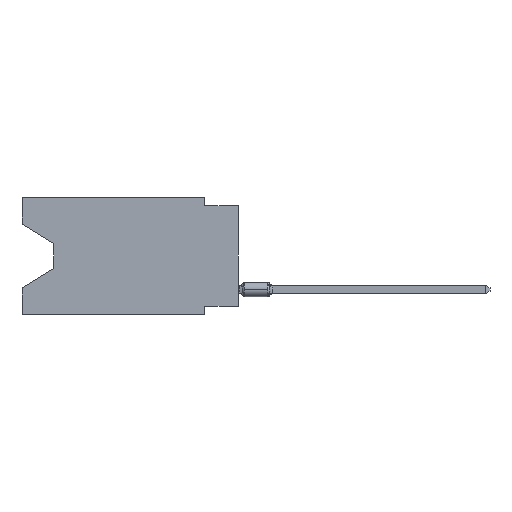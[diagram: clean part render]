
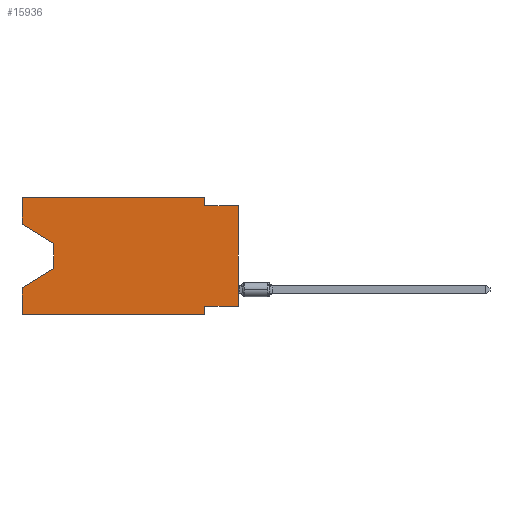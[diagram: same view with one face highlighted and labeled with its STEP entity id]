
A CAD part, left-side view. The second image highlights one B-rep face of the part: STEP entity #15936.
In plain terms, the highlighted planar face has unit normal (-1, 0, 0).
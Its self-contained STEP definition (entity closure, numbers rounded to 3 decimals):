
#45 = CARTESIAN_POINT ( 'NONE',  ( 0., 16.383, -8.89 ) ) ;
#59 = VECTOR ( 'NONE', #18303, 1000. ) ;
#830 = EDGE_CURVE ( 'NONE', #9263, #9711, #10362, .T. ) ;
#850 = LINE ( 'NONE', #15867, #10318 ) ;
#863 = VECTOR ( 'NONE', #14521, 1000. ) ;
#938 = VECTOR ( 'NONE', #13964, 1000. ) ;
#1732 = ORIENTED_EDGE ( 'NONE', *, *, #13332, .F. ) ;
#1753 = VERTEX_POINT ( 'NONE', #17822 ) ;
#1893 = VERTEX_POINT ( 'NONE', #14562 ) ;
#1903 = EDGE_CURVE ( 'NONE', #18999, #1893, #7029, .T. ) ;
#1999 = LINE ( 'NONE', #7998, #16949 ) ;
#2088 = LINE ( 'NONE', #8080, #59 ) ;
#2540 = DIRECTION ( 'NONE',  ( 0., 0., -1. ) ) ;
#2624 = CARTESIAN_POINT ( 'NONE',  ( 0., 0., -8.255 ) ) ;
#3233 = EDGE_LOOP ( 'NONE', ( #17978, #8627, #7239, #8827, #5678, #8044, #18217, #5854, #4483, #6046, #1732, #8704 ) ) ;
#4319 = CARTESIAN_POINT ( 'NONE',  ( 0., 13.97, -5.385 ) ) ;
#4483 = ORIENTED_EDGE ( 'NONE', *, *, #12300, .F. ) ;
#4683 = DIRECTION ( 'NONE',  ( 0., 0., 1. ) ) ;
#4895 = VERTEX_POINT ( 'NONE', #19130 ) ;
#4919 = VECTOR ( 'NONE', #6568, 1000. ) ;
#4926 = EDGE_CURVE ( 'NONE', #18999, #15049, #16763, .T. ) ;
#4992 = CARTESIAN_POINT ( 'NONE',  ( 0., 0., -0.635 ) ) ;
#5051 = LINE ( 'NONE', #5227, #938 ) ;
#5227 = CARTESIAN_POINT ( 'NONE',  ( 0., 2.54, 0. ) ) ;
#5397 = EDGE_CURVE ( 'NONE', #9263, #11819, #1999, .T. ) ;
#5626 = VERTEX_POINT ( 'NONE', #17776 ) ;
#5678 = ORIENTED_EDGE ( 'NONE', *, *, #4926, .T. ) ;
#5681 = VECTOR ( 'NONE', #16667, 1000. ) ;
#5854 = ORIENTED_EDGE ( 'NONE', *, *, #830, .T. ) ;
#6046 = ORIENTED_EDGE ( 'NONE', *, *, #9936, .F. ) ;
#6436 = DIRECTION ( 'NONE',  ( 0., 1., 0. ) ) ;
#6568 = DIRECTION ( 'NONE',  ( 0., -1., 0. ) ) ;
#6731 = DIRECTION ( 'NONE',  ( 0., 0., 1. ) ) ;
#7029 = LINE ( 'NONE', #9866, #13576 ) ;
#7239 = ORIENTED_EDGE ( 'NONE', *, *, #18160, .T. ) ;
#7241 = LINE ( 'NONE', #14965, #12222 ) ;
#7480 = AXIS2_PLACEMENT_3D ( 'NONE', #15069, #14025, #18013 ) ;
#7541 = CARTESIAN_POINT ( 'NONE',  ( 0., 16.383, 0. ) ) ;
#7979 = PLANE ( 'NONE',  #7480 ) ;
#7998 = CARTESIAN_POINT ( 'NONE',  ( 0., 0., -8.255 ) ) ;
#8044 = ORIENTED_EDGE ( 'NONE', *, *, #15213, .F. ) ;
#8080 = CARTESIAN_POINT ( 'NONE',  ( 0., 13.97, -3.505 ) ) ;
#8383 = VERTEX_POINT ( 'NONE', #12619 ) ;
#8545 = VECTOR ( 'NONE', #10458, 1000. ) ;
#8553 = LINE ( 'NONE', #13445, #863 ) ;
#8627 = ORIENTED_EDGE ( 'NONE', *, *, #19151, .T. ) ;
#8704 = ORIENTED_EDGE ( 'NONE', *, *, #9469, .F. ) ;
#8827 = ORIENTED_EDGE ( 'NONE', *, *, #1903, .F. ) ;
#8927 = DIRECTION ( 'NONE',  ( 0., 0.855, -0.519 ) ) ;
#9263 = VERTEX_POINT ( 'NONE', #2624 ) ;
#9469 = EDGE_CURVE ( 'NONE', #8383, #1753, #10583, .T. ) ;
#9711 = VERTEX_POINT ( 'NONE', #17412 ) ;
#9866 = CARTESIAN_POINT ( 'NONE',  ( 0., 16.383, 0. ) ) ;
#9896 = LINE ( 'NONE', #4992, #4919 ) ;
#9936 = EDGE_CURVE ( 'NONE', #18214, #4895, #5051, .T. ) ;
#10318 = VECTOR ( 'NONE', #2540, 1000. ) ;
#10362 = LINE ( 'NONE', #13372, #8545 ) ;
#10385 = DIRECTION ( 'NONE',  ( 0., -0.855, -0.519 ) ) ;
#10416 = LINE ( 'NONE', #16381, #18212 ) ;
#10458 = DIRECTION ( 'NONE',  ( 0., 0., 1. ) ) ;
#10583 = LINE ( 'NONE', #7541, #19101 ) ;
#11819 = VERTEX_POINT ( 'NONE', #18550 ) ;
#12222 = VECTOR ( 'NONE', #10385, 1000. ) ;
#12300 = EDGE_CURVE ( 'NONE', #4895, #9711, #9896, .T. ) ;
#12619 = CARTESIAN_POINT ( 'NONE',  ( 0., 16.383, -2.038 ) ) ;
#13332 = EDGE_CURVE ( 'NONE', #1753, #18214, #8553, .T. ) ;
#13372 = CARTESIAN_POINT ( 'NONE',  ( 0., 0., 0. ) ) ;
#13445 = CARTESIAN_POINT ( 'NONE',  ( 0., 16.383, 0. ) ) ;
#13576 = VECTOR ( 'NONE', #6731, 1000. ) ;
#13964 = DIRECTION ( 'NONE',  ( 0., 0., -1. ) ) ;
#14025 = DIRECTION ( 'NONE',  ( 1., 0., 0. ) ) ;
#14521 = DIRECTION ( 'NONE',  ( 0., -1., 0. ) ) ;
#14562 = CARTESIAN_POINT ( 'NONE',  ( 0., 16.383, -6.852 ) ) ;
#14965 = CARTESIAN_POINT ( 'NONE',  ( 0., 16.383, -2.038 ) ) ;
#15049 = VERTEX_POINT ( 'NONE', #16575 ) ;
#15069 = CARTESIAN_POINT ( 'NONE',  ( 0., 16.383, 0. ) ) ;
#15213 = EDGE_CURVE ( 'NONE', #11819, #15049, #850, .T. ) ;
#15867 = CARTESIAN_POINT ( 'NONE',  ( 0., 2.54, -8.89 ) ) ;
#15936 = ADVANCED_FACE ( 'NONE', ( #16521 ), #7979, .F. ) ;
#16381 = CARTESIAN_POINT ( 'NONE',  ( 0., 13.97, -5.385 ) ) ;
#16521 = FACE_OUTER_BOUND ( 'NONE', #3233, .T. ) ;
#16575 = CARTESIAN_POINT ( 'NONE',  ( 0., 2.54, -8.89 ) ) ;
#16667 = DIRECTION ( 'NONE',  ( 0., -1., 0. ) ) ;
#16763 = LINE ( 'NONE', #17954, #5681 ) ;
#16949 = VECTOR ( 'NONE', #6436, 1000. ) ;
#17116 = EDGE_CURVE ( 'NONE', #8383, #5626, #7241, .T. ) ;
#17412 = CARTESIAN_POINT ( 'NONE',  ( 0., 0., -0.635 ) ) ;
#17693 = VERTEX_POINT ( 'NONE', #4319 ) ;
#17776 = CARTESIAN_POINT ( 'NONE',  ( 0., 13.97, -3.505 ) ) ;
#17822 = CARTESIAN_POINT ( 'NONE',  ( 0., 16.383, 0. ) ) ;
#17954 = CARTESIAN_POINT ( 'NONE',  ( 0., 16.383, -8.89 ) ) ;
#17978 = ORIENTED_EDGE ( 'NONE', *, *, #17116, .T. ) ;
#18013 = DIRECTION ( 'NONE',  ( 0., 0., -1. ) ) ;
#18048 = CARTESIAN_POINT ( 'NONE',  ( 0., 2.54, 0. ) ) ;
#18160 = EDGE_CURVE ( 'NONE', #17693, #1893, #10416, .T. ) ;
#18212 = VECTOR ( 'NONE', #8927, 1000. ) ;
#18214 = VERTEX_POINT ( 'NONE', #18048 ) ;
#18217 = ORIENTED_EDGE ( 'NONE', *, *, #5397, .F. ) ;
#18303 = DIRECTION ( 'NONE',  ( 0., 0., -1. ) ) ;
#18550 = CARTESIAN_POINT ( 'NONE',  ( 0., 2.54, -8.255 ) ) ;
#18999 = VERTEX_POINT ( 'NONE', #45 ) ;
#19101 = VECTOR ( 'NONE', #4683, 1000. ) ;
#19130 = CARTESIAN_POINT ( 'NONE',  ( 0., 2.54, -0.635 ) ) ;
#19151 = EDGE_CURVE ( 'NONE', #5626, #17693, #2088, .T. ) ;
